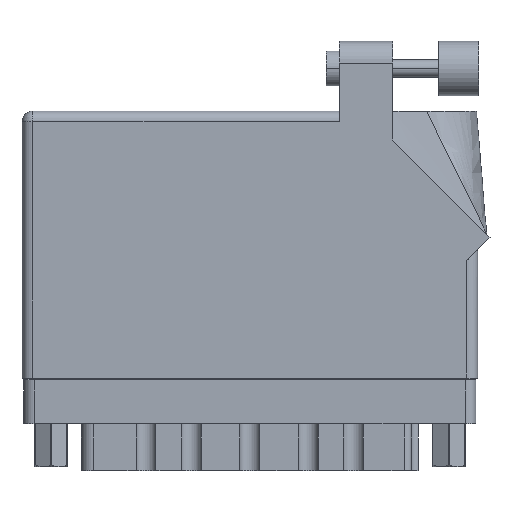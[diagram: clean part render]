
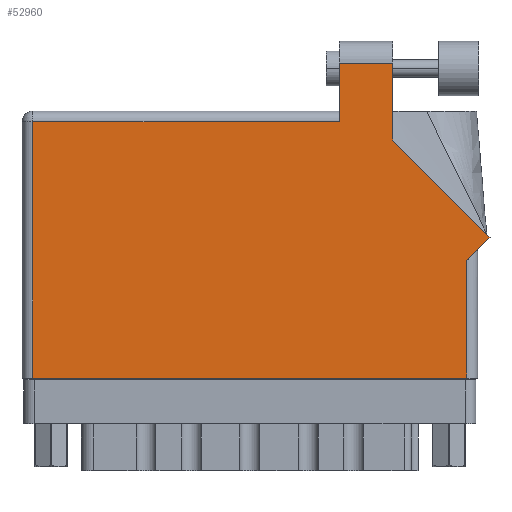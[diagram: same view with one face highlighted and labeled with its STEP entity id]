
A CAD part, front view. The second image highlights one B-rep face of the part: STEP entity #52960.
In plain terms, the highlighted face is planar.
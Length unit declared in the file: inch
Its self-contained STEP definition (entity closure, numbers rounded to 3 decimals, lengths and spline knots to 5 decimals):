
#164 = PLANE ( 'NONE',  #27590 ) ;
#188 = VECTOR ( 'NONE', #6156, 39.37008 ) ;
#535 = LINE ( 'NONE', #50724, #59953 ) ;
#2371 = CARTESIAN_POINT ( 'NONE',  ( 1.819, 1.805, 0. ) ) ;
#3180 = LINE ( 'NONE', #34720, #48258 ) ;
#5238 = CARTESIAN_POINT ( 'NONE',  ( 2.68271, 0.80771, 0. ) ) ;
#5247 = ORIENTED_EDGE ( 'NONE', *, *, #36907, .T. ) ;
#5554 = LINE ( 'NONE', #2371, #51465 ) ;
#6156 = DIRECTION ( 'NONE',  ( 1., 0., 0. ) ) ;
#6913 = VECTOR ( 'NONE', #49926, 39.37008 ) ;
#7060 = VERTEX_POINT ( 'NONE', #5238 ) ;
#7127 = VERTEX_POINT ( 'NONE', #10280 ) ;
#7537 = CARTESIAN_POINT ( 'NONE',  ( 2.126, 1.805, 0. ) ) ;
#9952 = CARTESIAN_POINT ( 'NONE',  ( 2.612, 0.737, 0. ) ) ;
#10280 = CARTESIAN_POINT ( 'NONE',  ( 2.55, 0.675, 0. ) ) ;
#11186 = CARTESIAN_POINT ( 'NONE',  ( 1.819, 1.468, 0. ) ) ;
#12551 = CARTESIAN_POINT ( 'NONE',  ( 0.062, 0., 0. ) ) ;
#12768 = VECTOR ( 'NONE', #22079, 39.37008 ) ;
#13526 = EDGE_CURVE ( 'NONE', #25524, #18914, #21118, .T. ) ;
#15121 = DIRECTION ( 'NONE',  ( -1., 0., 0. ) ) ;
#15656 = CARTESIAN_POINT ( 'NONE',  ( 0., 1.53, 0. ) ) ;
#16070 = DIRECTION ( 'NONE',  ( -0.707, 0.707, 0. ) ) ;
#16637 = VECTOR ( 'NONE', #18985, 39.37008 ) ;
#18914 = VERTEX_POINT ( 'NONE', #41981 ) ;
#18985 = DIRECTION ( 'NONE',  ( 0.707, 0.707, 0. ) ) ;
#19036 = ORIENTED_EDGE ( 'NONE', *, *, #33174, .T. ) ;
#21118 = LINE ( 'NONE', #44419, #188 ) ;
#22079 = DIRECTION ( 'NONE',  ( -1., 0., 0. ) ) ;
#25281 = FACE_OUTER_BOUND ( 'NONE', #38161, .T. ) ;
#25524 = VERTEX_POINT ( 'NONE', #56875 ) ;
#25531 = VERTEX_POINT ( 'NONE', #31138 ) ;
#26142 = CARTESIAN_POINT ( 'NONE',  ( 2.55, 0.737, 0. ) ) ;
#26775 = DIRECTION ( 'NONE',  ( 0., 1., 0. ) ) ;
#27590 = AXIS2_PLACEMENT_3D ( 'NONE', #15656, #37357, #15121 ) ;
#29055 = VECTOR ( 'NONE', #26775, 39.37008 ) ;
#31090 = DIRECTION ( 'NONE',  ( 0., -1., 0. ) ) ;
#31138 = CARTESIAN_POINT ( 'NONE',  ( 0.062, 1.468, 0. ) ) ;
#33117 = VERTEX_POINT ( 'NONE', #34707 ) ;
#33174 = EDGE_CURVE ( 'NONE', #51419, #43614, #54284, .T. ) ;
#33453 = ORIENTED_EDGE ( 'NONE', *, *, #39226, .T. ) ;
#34707 = CARTESIAN_POINT ( 'NONE',  ( 1.819, 1.805, 0. ) ) ;
#34720 = CARTESIAN_POINT ( 'NONE',  ( 2.68271, 0.80771, 0. ) ) ;
#36143 = ORIENTED_EDGE ( 'NONE', *, *, #13526, .T. ) ;
#36644 = DIRECTION ( 'NONE',  ( 0., -1., 0. ) ) ;
#36907 = EDGE_CURVE ( 'NONE', #18914, #7127, #39604, .T. ) ;
#37357 = DIRECTION ( 'NONE',  ( 0., 0., -1. ) ) ;
#37497 = ORIENTED_EDGE ( 'NONE', *, *, #49669, .T. ) ;
#38161 = EDGE_LOOP ( 'NONE', ( #19036, #33453, #45478, #46473, #46122, #36143, #5247, #40683, #37497 ) ) ;
#38182 = EDGE_CURVE ( 'NONE', #25531, #25524, #52741, .T. ) ;
#39226 = EDGE_CURVE ( 'NONE', #43614, #33117, #5554, .T. ) ;
#39604 = LINE ( 'NONE', #26142, #29055 ) ;
#40584 = EDGE_CURVE ( 'NONE', #7127, #7060, #53603, .T. ) ;
#40683 = ORIENTED_EDGE ( 'NONE', *, *, #40584, .T. ) ;
#41981 = CARTESIAN_POINT ( 'NONE',  ( 2.55, 0., 0. ) ) ;
#43141 = EDGE_CURVE ( 'NONE', #52914, #25531, #52645, .T. ) ;
#43614 = VERTEX_POINT ( 'NONE', #7537 ) ;
#44419 = CARTESIAN_POINT ( 'NONE',  ( 0., 0., 0. ) ) ;
#44831 = EDGE_CURVE ( 'NONE', #33117, #52914, #535, .T. ) ;
#45478 = ORIENTED_EDGE ( 'NONE', *, *, #44831, .T. ) ;
#46122 = ORIENTED_EDGE ( 'NONE', *, *, #38182, .T. ) ;
#46473 = ORIENTED_EDGE ( 'NONE', *, *, #43141, .T. ) ;
#48258 = VECTOR ( 'NONE', #16070, 39.37008 ) ;
#49669 = EDGE_CURVE ( 'NONE', #7060, #51419, #3180, .T. ) ;
#49926 = DIRECTION ( 'NONE',  ( 0., 1., 0. ) ) ;
#50079 = DIRECTION ( 'NONE',  ( -1., 0., 0. ) ) ;
#50724 = CARTESIAN_POINT ( 'NONE',  ( 1.819, 1.53, 0. ) ) ;
#51419 = VERTEX_POINT ( 'NONE', #57752 ) ;
#51465 = VECTOR ( 'NONE', #50079, 39.37008 ) ;
#52625 = VECTOR ( 'NONE', #36644, 39.37008 ) ;
#52645 = LINE ( 'NONE', #55714, #12768 ) ;
#52741 = LINE ( 'NONE', #12551, #52625 ) ;
#52914 = VERTEX_POINT ( 'NONE', #11186 ) ;
#52960 = ADVANCED_FACE ( 'NONE', ( #25281 ), #164, .F. ) ;
#53603 = LINE ( 'NONE', #9952, #16637 ) ;
#54284 = LINE ( 'NONE', #54547, #6913 ) ;
#54547 = CARTESIAN_POINT ( 'NONE',  ( 2.126, 1.36442, 0. ) ) ;
#55714 = CARTESIAN_POINT ( 'NONE',  ( 0., 1.468, 0. ) ) ;
#56875 = CARTESIAN_POINT ( 'NONE',  ( 0.062, 0., 0. ) ) ;
#57752 = CARTESIAN_POINT ( 'NONE',  ( 2.126, 1.36442, 0. ) ) ;
#59953 = VECTOR ( 'NONE', #31090, 39.37008 ) ;
